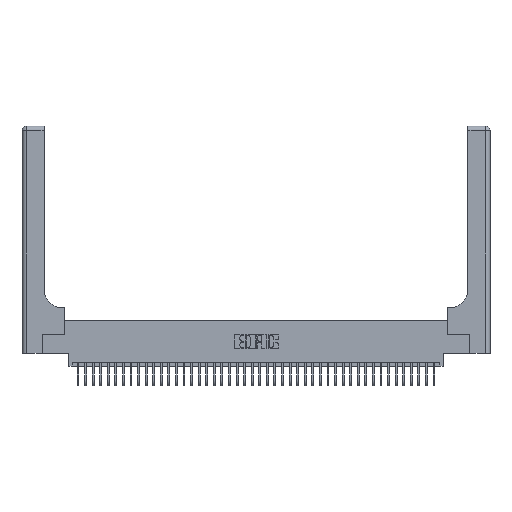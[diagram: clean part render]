
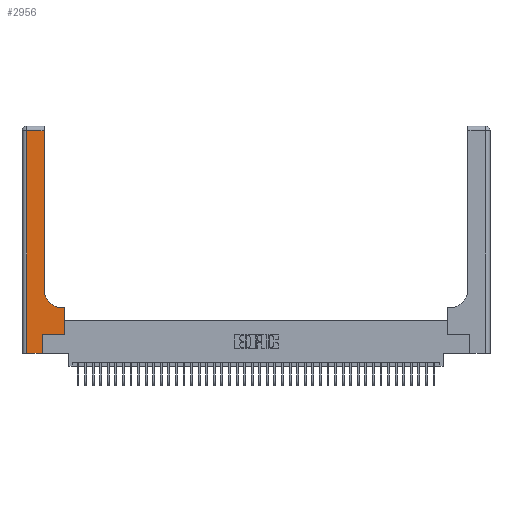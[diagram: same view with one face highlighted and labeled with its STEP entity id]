
A CAD part, top view. The second image highlights one B-rep face of the part: STEP entity #2956.
In plain terms, the highlighted planar face has unit normal (0, 0, 1).
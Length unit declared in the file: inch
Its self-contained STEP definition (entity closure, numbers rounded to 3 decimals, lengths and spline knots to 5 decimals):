
#228 = LINE ( 'NONE', #38995, #35273 ) ;
#2777 = ORIENTED_EDGE ( 'NONE', *, *, #11714, .T. ) ;
#2956 = ADVANCED_FACE ( 'NONE', ( #37555 ), #33373, .F. ) ;
#5019 = DIRECTION ( 'NONE',  ( 0., 1., 0. ) ) ;
#5173 = CARTESIAN_POINT ( 'NONE',  ( 0.5585, 0.25, 0.37 ) ) ;
#5264 = DIRECTION ( 'NONE',  ( 0., 1., 0. ) ) ;
#7003 = ORIENTED_EDGE ( 'NONE', *, *, #40585, .T. ) ;
#7555 = ORIENTED_EDGE ( 'NONE', *, *, #8134, .T. ) ;
#7649 = ORIENTED_EDGE ( 'NONE', *, *, #40721, .T. ) ;
#8134 = EDGE_CURVE ( 'NONE', #14090, #9413, #33959, .T. ) ;
#9383 = VERTEX_POINT ( 'NONE', #13313 ) ;
#9413 = VERTEX_POINT ( 'NONE', #23623 ) ;
#9601 = VECTOR ( 'NONE', #9619, 39.37008 ) ;
#9619 = DIRECTION ( 'NONE',  ( -1., 0., 0. ) ) ;
#9733 = VECTOR ( 'NONE', #10577, 39.37008 ) ;
#10286 = CARTESIAN_POINT ( 'NONE',  ( 0.2915, 0.85, 0.37 ) ) ;
#10313 = VERTEX_POINT ( 'NONE', #10286 ) ;
#10577 = DIRECTION ( 'NONE',  ( 0., -1., 0. ) ) ;
#11355 = DIRECTION ( 'NONE',  ( -1., 0., 0. ) ) ;
#11634 = DIRECTION ( 'NONE',  ( 1., 0., 0. ) ) ;
#11714 = EDGE_CURVE ( 'NONE', #16569, #20443, #34031, .T. ) ;
#12856 = AXIS2_PLACEMENT_3D ( 'NONE', #37522, #17336, #40899 ) ;
#13313 = CARTESIAN_POINT ( 'NONE',  ( 0.06, 2.94, 0.37 ) ) ;
#14090 = VERTEX_POINT ( 'NONE', #5173 ) ;
#14619 = DIRECTION ( 'NONE',  ( 1., 0., 0. ) ) ;
#15019 = ORIENTED_EDGE ( 'NONE', *, *, #18329, .T. ) ;
#15334 = CARTESIAN_POINT ( 'NONE',  ( 0.269, 0., 0.37 ) ) ;
#16569 = VERTEX_POINT ( 'NONE', #20764 ) ;
#17336 = DIRECTION ( 'NONE',  ( 0., 0., -1. ) ) ;
#17968 = VECTOR ( 'NONE', #5019, 39.37008 ) ;
#18329 = EDGE_CURVE ( 'NONE', #9383, #16569, #19779, .T. ) ;
#19409 = CARTESIAN_POINT ( 'NONE',  ( 0.2915, 2.94, 0.37 ) ) ;
#19750 = EDGE_CURVE ( 'NONE', #24305, #9383, #28600, .T. ) ;
#19779 = LINE ( 'NONE', #23999, #9733 ) ;
#19934 = DIRECTION ( 'NONE',  ( 0., 0., -1. ) ) ;
#20443 = VERTEX_POINT ( 'NONE', #33344 ) ;
#20764 = CARTESIAN_POINT ( 'NONE',  ( 0.06, 0., 0.37 ) ) ;
#20774 = ORIENTED_EDGE ( 'NONE', *, *, #19750, .T. ) ;
#21215 = EDGE_LOOP ( 'NONE', ( #21265, #20774, #15019, #2777, #7649, #7003, #7555, #35602, #23978 ) ) ;
#21265 = ORIENTED_EDGE ( 'NONE', *, *, #24781, .T. ) ;
#23111 = DIRECTION ( 'NONE',  ( 0., 1., 0. ) ) ;
#23623 = CARTESIAN_POINT ( 'NONE',  ( 0.5585, 0.6, 0.37 ) ) ;
#23978 = ORIENTED_EDGE ( 'NONE', *, *, #43677, .T. ) ;
#23999 = CARTESIAN_POINT ( 'NONE',  ( 0.06, 3., 0.37 ) ) ;
#24291 = VECTOR ( 'NONE', #14619, 39.37008 ) ;
#24305 = VERTEX_POINT ( 'NONE', #19409 ) ;
#24781 = EDGE_CURVE ( 'NONE', #10313, #24305, #228, .T. ) ;
#25464 = VERTEX_POINT ( 'NONE', #32320 ) ;
#25764 = VECTOR ( 'NONE', #11355, 39.37008 ) ;
#26454 = CARTESIAN_POINT ( 'NONE',  ( 0., 2.94, 0.37 ) ) ;
#26581 = CARTESIAN_POINT ( 'NONE',  ( 0., 3., 0.37 ) ) ;
#28443 = CARTESIAN_POINT ( 'NONE',  ( 0., 0., 0.37 ) ) ;
#28600 = LINE ( 'NONE', #26454, #9601 ) ;
#29450 = AXIS2_PLACEMENT_3D ( 'NONE', #26581, #19934, #43492 ) ;
#31746 = CIRCLE ( 'NONE', #12856, 0.25 ) ;
#31761 = EDGE_CURVE ( 'NONE', #9413, #25464, #34742, .T. ) ;
#31820 = VECTOR ( 'NONE', #23111, 39.37008 ) ;
#32320 = CARTESIAN_POINT ( 'NONE',  ( 0.5415, 0.6, 0.37 ) ) ;
#33202 = CARTESIAN_POINT ( 'NONE',  ( 0.5585, 0.25, 0.37 ) ) ;
#33301 = LINE ( 'NONE', #34797, #24291 ) ;
#33344 = CARTESIAN_POINT ( 'NONE',  ( 0.269, 0., 0.37 ) ) ;
#33373 = PLANE ( 'NONE',  #29450 ) ;
#33959 = LINE ( 'NONE', #33202, #31820 ) ;
#34031 = LINE ( 'NONE', #28443, #41436 ) ;
#34498 = VERTEX_POINT ( 'NONE', #41832 ) ;
#34742 = LINE ( 'NONE', #38344, #25764 ) ;
#34797 = CARTESIAN_POINT ( 'NONE',  ( 0.269, 0.25, 0.37 ) ) ;
#35273 = VECTOR ( 'NONE', #5264, 39.37008 ) ;
#35602 = ORIENTED_EDGE ( 'NONE', *, *, #31761, .T. ) ;
#37522 = CARTESIAN_POINT ( 'NONE',  ( 0.5415, 0.85, 0.37 ) ) ;
#37555 = FACE_OUTER_BOUND ( 'NONE', #21215, .T. ) ;
#38344 = CARTESIAN_POINT ( 'NONE',  ( 0.2915, 0.6, 0.37 ) ) ;
#38995 = CARTESIAN_POINT ( 'NONE',  ( 0.2915, 3., 0.37 ) ) ;
#39071 = LINE ( 'NONE', #15334, #17968 ) ;
#40585 = EDGE_CURVE ( 'NONE', #34498, #14090, #33301, .T. ) ;
#40721 = EDGE_CURVE ( 'NONE', #20443, #34498, #39071, .T. ) ;
#40899 = DIRECTION ( 'NONE',  ( 1., 0., 0. ) ) ;
#41436 = VECTOR ( 'NONE', #11634, 39.37008 ) ;
#41832 = CARTESIAN_POINT ( 'NONE',  ( 0.269, 0.25, 0.37 ) ) ;
#43492 = DIRECTION ( 'NONE',  ( -1., 0., 0. ) ) ;
#43677 = EDGE_CURVE ( 'NONE', #25464, #10313, #31746, .T. ) ;
